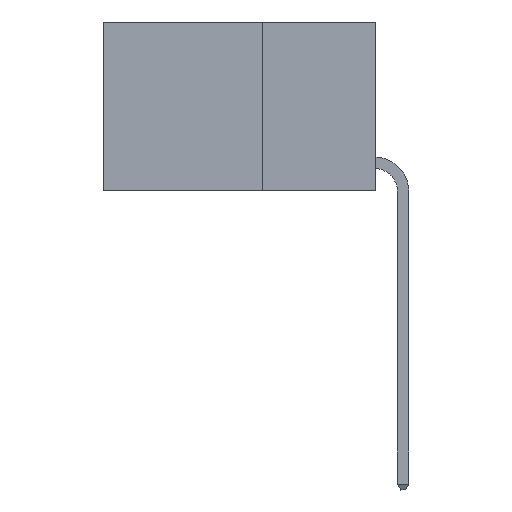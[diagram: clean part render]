
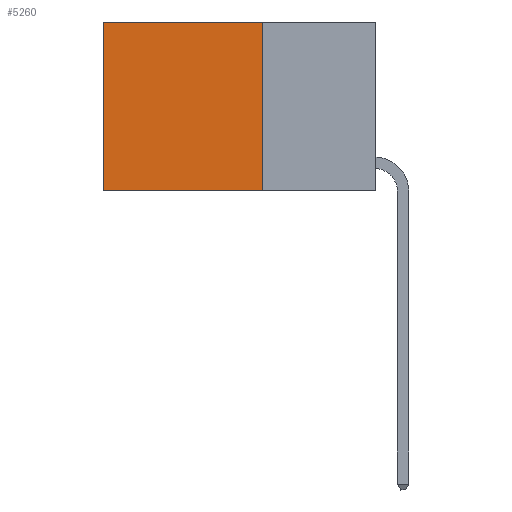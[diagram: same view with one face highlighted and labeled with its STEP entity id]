
A CAD part, left-side view. The second image highlights one B-rep face of the part: STEP entity #5260.
In plain terms, the highlighted planar face has unit normal (-1, 0, 0).
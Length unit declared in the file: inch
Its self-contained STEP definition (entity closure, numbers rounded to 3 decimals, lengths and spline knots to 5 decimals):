
#324 = VERTEX_POINT ( 'NONE', #12547 ) ;
#540 = DIRECTION ( 'NONE',  ( 0., 1., 0. ) ) ;
#1730 = DIRECTION ( 'NONE',  ( 1., 0., 0. ) ) ;
#1812 = PLANE ( 'NONE',  #2808 ) ;
#2134 = VECTOR ( 'NONE', #2491, 39.37008 ) ;
#2237 = VERTEX_POINT ( 'NONE', #4010 ) ;
#2491 = DIRECTION ( 'NONE',  ( 0., 0., -1. ) ) ;
#2808 = AXIS2_PLACEMENT_3D ( 'NONE', #12682, #1730, #7172 ) ;
#3191 = CARTESIAN_POINT ( 'NONE',  ( 0.2625, 0.25, 0. ) ) ;
#3834 = CARTESIAN_POINT ( 'NONE',  ( 0.2625, 0.25, 0. ) ) ;
#4010 = CARTESIAN_POINT ( 'NONE',  ( 0.2625, 0.25, -0.37 ) ) ;
#4143 = VERTEX_POINT ( 'NONE', #15948 ) ;
#5033 = VECTOR ( 'NONE', #540, 39.37008 ) ;
#5042 = LINE ( 'NONE', #10476, #17224 ) ;
#5050 = ORIENTED_EDGE ( 'NONE', *, *, #15523, .F. ) ;
#5260 = ADVANCED_FACE ( 'NONE', ( #8586 ), #1812, .F. ) ;
#6094 = VECTOR ( 'NONE', #10300, 39.37008 ) ;
#7172 = DIRECTION ( 'NONE',  ( 0., 0., -1. ) ) ;
#7314 = LINE ( 'NONE', #15609, #5033 ) ;
#7617 = ORIENTED_EDGE ( 'NONE', *, *, #12727, .T. ) ;
#8586 = FACE_OUTER_BOUND ( 'NONE', #12726, .T. ) ;
#10300 = DIRECTION ( 'NONE',  ( 0., 0., -1. ) ) ;
#10476 = CARTESIAN_POINT ( 'NONE',  ( 0.2625, 0.25, -0.37 ) ) ;
#12547 = CARTESIAN_POINT ( 'NONE',  ( 0.2625, 0.6, 0. ) ) ;
#12682 = CARTESIAN_POINT ( 'NONE',  ( 0.2625, 0.25, 0. ) ) ;
#12726 = EDGE_LOOP ( 'NONE', ( #7617, #5050, #15185, #13652 ) ) ;
#12727 = EDGE_CURVE ( 'NONE', #324, #4143, #15836, .T. ) ;
#13652 = ORIENTED_EDGE ( 'NONE', *, *, #16649, .T. ) ;
#14024 = VERTEX_POINT ( 'NONE', #3191 ) ;
#15185 = ORIENTED_EDGE ( 'NONE', *, *, #16303, .F. ) ;
#15523 = EDGE_CURVE ( 'NONE', #2237, #4143, #5042, .T. ) ;
#15609 = CARTESIAN_POINT ( 'NONE',  ( 0.2625, 0.25, 0. ) ) ;
#15836 = LINE ( 'NONE', #17083, #6094 ) ;
#15881 = LINE ( 'NONE', #3834, #2134 ) ;
#15932 = DIRECTION ( 'NONE',  ( 0., 1., 0. ) ) ;
#15948 = CARTESIAN_POINT ( 'NONE',  ( 0.2625, 0.6, -0.37 ) ) ;
#16303 = EDGE_CURVE ( 'NONE', #14024, #2237, #15881, .T. ) ;
#16649 = EDGE_CURVE ( 'NONE', #14024, #324, #7314, .T. ) ;
#17083 = CARTESIAN_POINT ( 'NONE',  ( 0.2625, 0.6, 0. ) ) ;
#17224 = VECTOR ( 'NONE', #15932, 39.37008 ) ;
